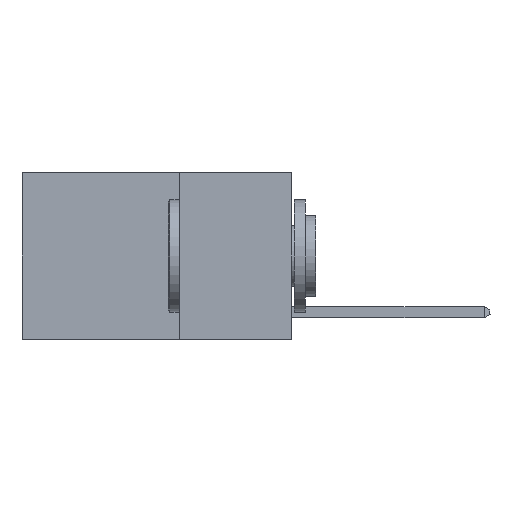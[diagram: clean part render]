
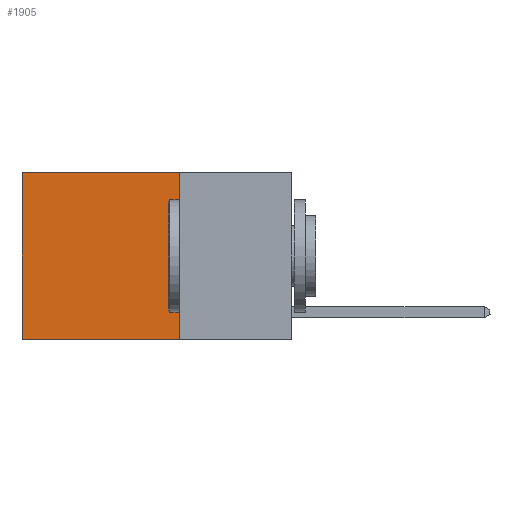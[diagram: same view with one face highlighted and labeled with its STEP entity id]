
A CAD part, left-side view. The second image highlights one B-rep face of the part: STEP entity #1905.
In plain terms, the highlighted planar face has unit normal (-1, 0, 0).
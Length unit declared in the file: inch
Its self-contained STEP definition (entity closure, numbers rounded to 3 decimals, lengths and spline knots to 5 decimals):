
#81 = VECTOR ( 'NONE', #15370, 39.37008 ) ;
#85 = EDGE_CURVE ( 'NONE', #25017, #1644, #7983, .T. ) ;
#344 = DIRECTION ( 'NONE',  ( 0., 0., -1. ) ) ;
#1335 = CARTESIAN_POINT ( 'NONE',  ( 0.2625, 0.6, 0. ) ) ;
#1644 = VERTEX_POINT ( 'NONE', #11798 ) ;
#1905 = ADVANCED_FACE ( 'NONE', ( #7517 ), #13367, .F. ) ;
#2220 = DIRECTION ( 'NONE',  ( 1., 0., 0. ) ) ;
#4614 = EDGE_LOOP ( 'NONE', ( #24045, #5734, #18926, #22348 ) ) ;
#4768 = VECTOR ( 'NONE', #13150, 39.37008 ) ;
#5101 = EDGE_CURVE ( 'NONE', #22387, #19523, #19890, .T. ) ;
#5734 = ORIENTED_EDGE ( 'NONE', *, *, #11031, .F. ) ;
#6982 = VECTOR ( 'NONE', #344, 39.37008 ) ;
#7158 = AXIS2_PLACEMENT_3D ( 'NONE', #21152, #2220, #16002 ) ;
#7517 = FACE_OUTER_BOUND ( 'NONE', #4614, .T. ) ;
#7983 = LINE ( 'NONE', #15620, #81 ) ;
#9722 = CARTESIAN_POINT ( 'NONE',  ( 0.2625, 0.25, -0.37 ) ) ;
#11031 = EDGE_CURVE ( 'NONE', #19523, #1644, #24223, .T. ) ;
#11798 = CARTESIAN_POINT ( 'NONE',  ( 0.2625, 0.6, -0.37 ) ) ;
#12615 = EDGE_CURVE ( 'NONE', #22387, #25017, #20803, .T. ) ;
#13150 = DIRECTION ( 'NONE',  ( 0., 1., 0. ) ) ;
#13367 = PLANE ( 'NONE',  #7158 ) ;
#15168 = CARTESIAN_POINT ( 'NONE',  ( 0.2625, 0.25, 0. ) ) ;
#15370 = DIRECTION ( 'NONE',  ( 0., 0., -1. ) ) ;
#15620 = CARTESIAN_POINT ( 'NONE',  ( 0.2625, 0.6, 0. ) ) ;
#16002 = DIRECTION ( 'NONE',  ( 0., 0., -1. ) ) ;
#16340 = CARTESIAN_POINT ( 'NONE',  ( 0.2625, 0.25, 0. ) ) ;
#17874 = DIRECTION ( 'NONE',  ( 0., 1., 0. ) ) ;
#18926 = ORIENTED_EDGE ( 'NONE', *, *, #5101, .F. ) ;
#19523 = VERTEX_POINT ( 'NONE', #9722 ) ;
#19676 = VECTOR ( 'NONE', #17874, 39.37008 ) ;
#19890 = LINE ( 'NONE', #24182, #6982 ) ;
#20168 = CARTESIAN_POINT ( 'NONE',  ( 0.2625, 0.25, -0.37 ) ) ;
#20803 = LINE ( 'NONE', #15168, #4768 ) ;
#21152 = CARTESIAN_POINT ( 'NONE',  ( 0.2625, 0.25, 0. ) ) ;
#22348 = ORIENTED_EDGE ( 'NONE', *, *, #12615, .T. ) ;
#22387 = VERTEX_POINT ( 'NONE', #16340 ) ;
#24045 = ORIENTED_EDGE ( 'NONE', *, *, #85, .T. ) ;
#24182 = CARTESIAN_POINT ( 'NONE',  ( 0.2625, 0.25, 0. ) ) ;
#24223 = LINE ( 'NONE', #20168, #19676 ) ;
#25017 = VERTEX_POINT ( 'NONE', #1335 ) ;
